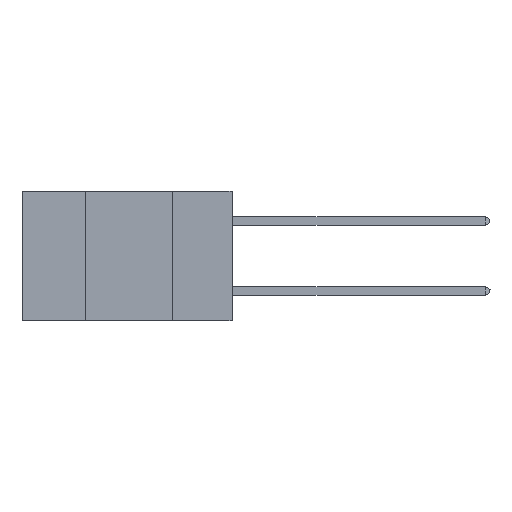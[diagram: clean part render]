
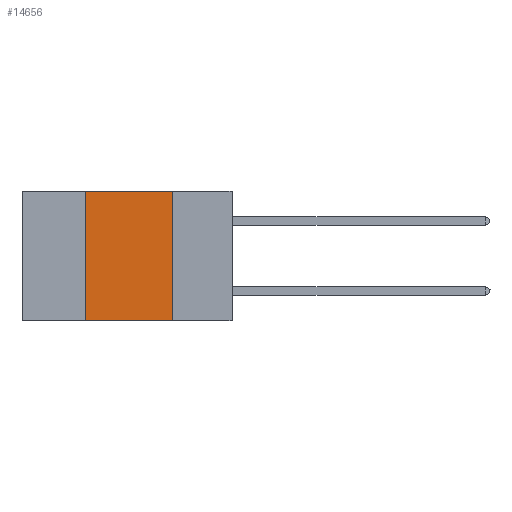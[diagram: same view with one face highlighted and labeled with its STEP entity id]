
A CAD part, left-side view. The second image highlights one B-rep face of the part: STEP entity #14656.
In plain terms, the highlighted planar face has unit normal (-1, 0, 0).
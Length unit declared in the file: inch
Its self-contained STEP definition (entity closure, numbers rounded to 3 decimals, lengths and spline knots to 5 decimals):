
#542 = DIRECTION ( 'NONE',  ( 0., -1., 0. ) ) ;
#2383 = VECTOR ( 'NONE', #32815, 39.37008 ) ;
#2822 = VERTEX_POINT ( 'NONE', #10808 ) ;
#3181 = LINE ( 'NONE', #4643, #31728 ) ;
#3734 = PLANE ( 'NONE',  #11195 ) ;
#4643 = CARTESIAN_POINT ( 'NONE',  ( 0., 0.42, 0. ) ) ;
#6041 = VECTOR ( 'NONE', #29434, 39.37008 ) ;
#6108 = VECTOR ( 'NONE', #542, 39.37008 ) ;
#7080 = DIRECTION ( 'NONE',  ( 1., 0., 0. ) ) ;
#7715 = VERTEX_POINT ( 'NONE', #23546 ) ;
#8936 = CARTESIAN_POINT ( 'NONE',  ( 0., 0.6, 0. ) ) ;
#8963 = ORIENTED_EDGE ( 'NONE', *, *, #34935, .F. ) ;
#10009 = EDGE_CURVE ( 'NONE', #2822, #26357, #24690, .T. ) ;
#10808 = CARTESIAN_POINT ( 'NONE',  ( 0., 0.42, -0.37 ) ) ;
#11195 = AXIS2_PLACEMENT_3D ( 'NONE', #15366, #7080, #23673 ) ;
#14656 = ADVANCED_FACE ( 'NONE', ( #21732 ), #3734, .F. ) ;
#15366 = CARTESIAN_POINT ( 'NONE',  ( 0., 0.6, 0. ) ) ;
#17670 = LINE ( 'NONE', #35147, #6041 ) ;
#17781 = EDGE_CURVE ( 'NONE', #2822, #7715, #3181, .T. ) ;
#18137 = ORIENTED_EDGE ( 'NONE', *, *, #17781, .F. ) ;
#21732 = FACE_OUTER_BOUND ( 'NONE', #22766, .T. ) ;
#21852 = CARTESIAN_POINT ( 'NONE',  ( 0., 0.17, 0. ) ) ;
#21858 = DIRECTION ( 'NONE',  ( 0., 0., 1. ) ) ;
#22766 = EDGE_LOOP ( 'NONE', ( #29116, #8963, #18137, #27088 ) ) ;
#23546 = CARTESIAN_POINT ( 'NONE',  ( 0., 0.42, 0. ) ) ;
#23673 = DIRECTION ( 'NONE',  ( 0., 0., -1. ) ) ;
#24317 = EDGE_CURVE ( 'NONE', #32305, #26357, #17670, .T. ) ;
#24690 = LINE ( 'NONE', #28629, #2383 ) ;
#26357 = VERTEX_POINT ( 'NONE', #31287 ) ;
#27088 = ORIENTED_EDGE ( 'NONE', *, *, #10009, .T. ) ;
#28629 = CARTESIAN_POINT ( 'NONE',  ( 0., 0.6, -0.37 ) ) ;
#29116 = ORIENTED_EDGE ( 'NONE', *, *, #24317, .F. ) ;
#29434 = DIRECTION ( 'NONE',  ( 0., 0., -1. ) ) ;
#31287 = CARTESIAN_POINT ( 'NONE',  ( 0., 0.17, -0.37 ) ) ;
#31728 = VECTOR ( 'NONE', #21858, 39.37008 ) ;
#32305 = VERTEX_POINT ( 'NONE', #21852 ) ;
#32815 = DIRECTION ( 'NONE',  ( 0., -1., 0. ) ) ;
#34243 = LINE ( 'NONE', #8936, #6108 ) ;
#34935 = EDGE_CURVE ( 'NONE', #7715, #32305, #34243, .T. ) ;
#35147 = CARTESIAN_POINT ( 'NONE',  ( 0., 0.17, 0. ) ) ;
